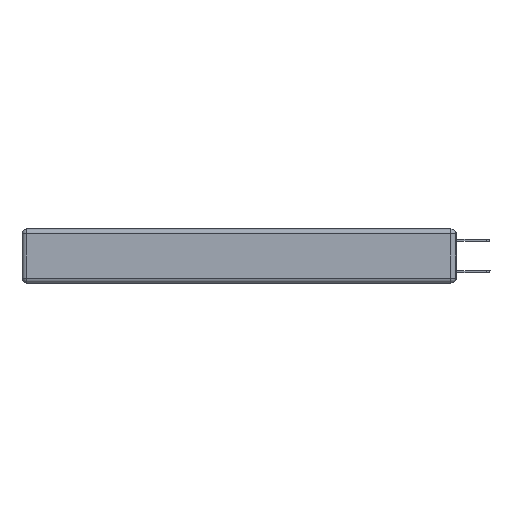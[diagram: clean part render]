
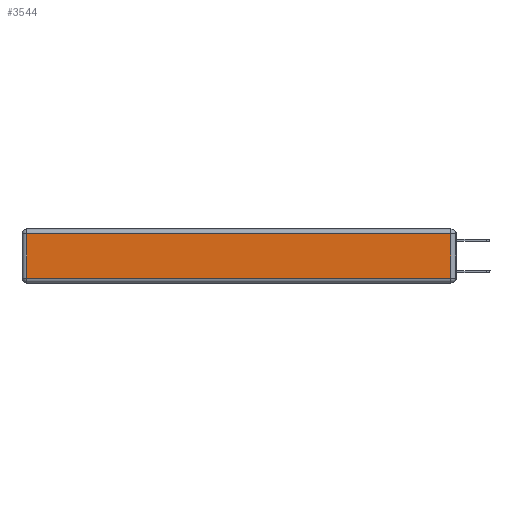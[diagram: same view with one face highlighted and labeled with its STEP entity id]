
A CAD part, left-side view. The second image highlights one B-rep face of the part: STEP entity #3544.
In plain terms, the highlighted planar face has unit normal (-1, 0, 0).
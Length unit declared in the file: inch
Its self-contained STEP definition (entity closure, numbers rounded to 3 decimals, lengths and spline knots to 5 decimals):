
#438 = DIRECTION ( 'NONE',  ( 0., 1., 0. ) ) ;
#695 = ORIENTED_EDGE ( 'NONE', *, *, #2584, .T. ) ;
#2058 = VERTEX_POINT ( 'NONE', #13453 ) ;
#2584 = EDGE_CURVE ( 'NONE', #12632, #4071, #16550, .T. ) ;
#2982 = DIRECTION ( 'NONE',  ( 0., 0., -1. ) ) ;
#3431 = CARTESIAN_POINT ( 'NONE',  ( 0., 0.03, -0.03 ) ) ;
#3544 = ADVANCED_FACE ( 'NONE', ( #15592 ), #6325, .T. ) ;
#3707 = DIRECTION ( 'NONE',  ( 0., 0., 1. ) ) ;
#3789 = CARTESIAN_POINT ( 'NONE',  ( 0., 0.03, -0.313 ) ) ;
#3906 = EDGE_CURVE ( 'NONE', #4071, #4980, #15319, .T. ) ;
#4071 = VERTEX_POINT ( 'NONE', #3431 ) ;
#4464 = LINE ( 'NONE', #12433, #13388 ) ;
#4932 = CARTESIAN_POINT ( 'NONE',  ( 0., 0., -0.343 ) ) ;
#4947 = ORIENTED_EDGE ( 'NONE', *, *, #3906, .T. ) ;
#4980 = VERTEX_POINT ( 'NONE', #14069 ) ;
#6325 = PLANE ( 'NONE',  #7503 ) ;
#7201 = LINE ( 'NONE', #12961, #13133 ) ;
#7503 = AXIS2_PLACEMENT_3D ( 'NONE', #4932, #10320, #3707 ) ;
#7961 = VECTOR ( 'NONE', #438, 39.37008 ) ;
#8337 = CARTESIAN_POINT ( 'NONE',  ( 0., 2.75, -0.03 ) ) ;
#9879 = DIRECTION ( 'NONE',  ( 0., 0., 1. ) ) ;
#10320 = DIRECTION ( 'NONE',  ( -1., 0., 0. ) ) ;
#11176 = CARTESIAN_POINT ( 'NONE',  ( 0., 0.03, -0.343 ) ) ;
#12272 = VECTOR ( 'NONE', #9879, 39.37008 ) ;
#12433 = CARTESIAN_POINT ( 'NONE',  ( 0., 2.72, -0.343 ) ) ;
#12632 = VERTEX_POINT ( 'NONE', #3789 ) ;
#12961 = CARTESIAN_POINT ( 'NONE',  ( 0., 0., -0.313 ) ) ;
#13133 = VECTOR ( 'NONE', #16785, 39.37008 ) ;
#13147 = ORIENTED_EDGE ( 'NONE', *, *, #16900, .T. ) ;
#13388 = VECTOR ( 'NONE', #2982, 39.37008 ) ;
#13453 = CARTESIAN_POINT ( 'NONE',  ( 0., 2.72, -0.313 ) ) ;
#14069 = CARTESIAN_POINT ( 'NONE',  ( 0., 2.72, -0.03 ) ) ;
#14458 = ORIENTED_EDGE ( 'NONE', *, *, #15868, .T. ) ;
#15319 = LINE ( 'NONE', #8337, #7961 ) ;
#15386 = EDGE_LOOP ( 'NONE', ( #13147, #695, #4947, #14458 ) ) ;
#15592 = FACE_OUTER_BOUND ( 'NONE', #15386, .T. ) ;
#15868 = EDGE_CURVE ( 'NONE', #4980, #2058, #4464, .T. ) ;
#16550 = LINE ( 'NONE', #11176, #12272 ) ;
#16785 = DIRECTION ( 'NONE',  ( 0., -1., 0. ) ) ;
#16900 = EDGE_CURVE ( 'NONE', #2058, #12632, #7201, .T. ) ;
